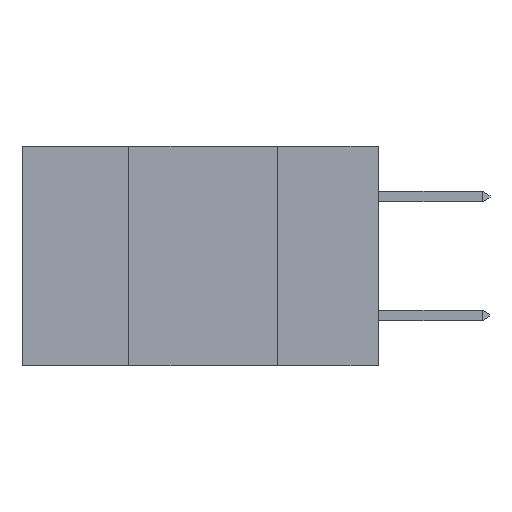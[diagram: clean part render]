
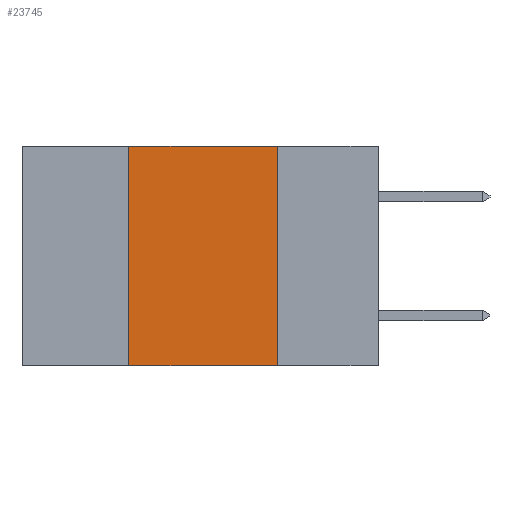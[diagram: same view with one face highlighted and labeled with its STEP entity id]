
A CAD part, left-side view. The second image highlights one B-rep face of the part: STEP entity #23745.
In plain terms, the highlighted planar face has unit normal (-1, 0, 0).
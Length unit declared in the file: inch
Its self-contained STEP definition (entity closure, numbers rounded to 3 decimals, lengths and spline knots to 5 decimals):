
#1469 = CARTESIAN_POINT ( 'NONE',  ( 0., 0.42, -0.37 ) ) ;
#1779 = AXIS2_PLACEMENT_3D ( 'NONE', #11722, #19130, #7992 ) ;
#1848 = FACE_OUTER_BOUND ( 'NONE', #9196, .T. ) ;
#2026 = DIRECTION ( 'NONE',  ( 0., 0., -1. ) ) ;
#2381 = ORIENTED_EDGE ( 'NONE', *, *, #21234, .F. ) ;
#3177 = LINE ( 'NONE', #22622, #22232 ) ;
#5093 = VECTOR ( 'NONE', #17527, 39.37008 ) ;
#5606 = VERTEX_POINT ( 'NONE', #1469 ) ;
#6128 = PLANE ( 'NONE',  #1779 ) ;
#6613 = CARTESIAN_POINT ( 'NONE',  ( 0., 0.42, 0. ) ) ;
#7143 = LINE ( 'NONE', #13176, #12174 ) ;
#7182 = VERTEX_POINT ( 'NONE', #6613 ) ;
#7631 = ORIENTED_EDGE ( 'NONE', *, *, #8282, .T. ) ;
#7992 = DIRECTION ( 'NONE',  ( 0., 0., -1. ) ) ;
#8282 = EDGE_CURVE ( 'NONE', #5606, #22634, #23363, .T. ) ;
#9196 = EDGE_LOOP ( 'NONE', ( #19017, #2381, #16993, #7631 ) ) ;
#9540 = EDGE_CURVE ( 'NONE', #5606, #7182, #3177, .T. ) ;
#9886 = CARTESIAN_POINT ( 'NONE',  ( 0., 0.6, -0.37 ) ) ;
#10079 = CARTESIAN_POINT ( 'NONE',  ( 0., 0.6, 0. ) ) ;
#10521 = CARTESIAN_POINT ( 'NONE',  ( 0., 0.17, -0.37 ) ) ;
#11722 = CARTESIAN_POINT ( 'NONE',  ( 0., 0.6, 0. ) ) ;
#11752 = DIRECTION ( 'NONE',  ( 0., 0., 1. ) ) ;
#11970 = CARTESIAN_POINT ( 'NONE',  ( 0., 0.17, 0. ) ) ;
#12088 = EDGE_CURVE ( 'NONE', #12834, #22634, #7143, .T. ) ;
#12174 = VECTOR ( 'NONE', #2026, 39.37008 ) ;
#12834 = VERTEX_POINT ( 'NONE', #11970 ) ;
#13176 = CARTESIAN_POINT ( 'NONE',  ( 0., 0.17, 0. ) ) ;
#13738 = VECTOR ( 'NONE', #20943, 39.37008 ) ;
#15016 = LINE ( 'NONE', #10079, #5093 ) ;
#16993 = ORIENTED_EDGE ( 'NONE', *, *, #9540, .F. ) ;
#17527 = DIRECTION ( 'NONE',  ( 0., -1., 0. ) ) ;
#19017 = ORIENTED_EDGE ( 'NONE', *, *, #12088, .F. ) ;
#19130 = DIRECTION ( 'NONE',  ( 1., 0., 0. ) ) ;
#20943 = DIRECTION ( 'NONE',  ( 0., -1., 0. ) ) ;
#21234 = EDGE_CURVE ( 'NONE', #7182, #12834, #15016, .T. ) ;
#22232 = VECTOR ( 'NONE', #11752, 39.37008 ) ;
#22622 = CARTESIAN_POINT ( 'NONE',  ( 0., 0.42, 0. ) ) ;
#22634 = VERTEX_POINT ( 'NONE', #10521 ) ;
#23363 = LINE ( 'NONE', #9886, #13738 ) ;
#23745 = ADVANCED_FACE ( 'NONE', ( #1848 ), #6128, .F. ) ;
